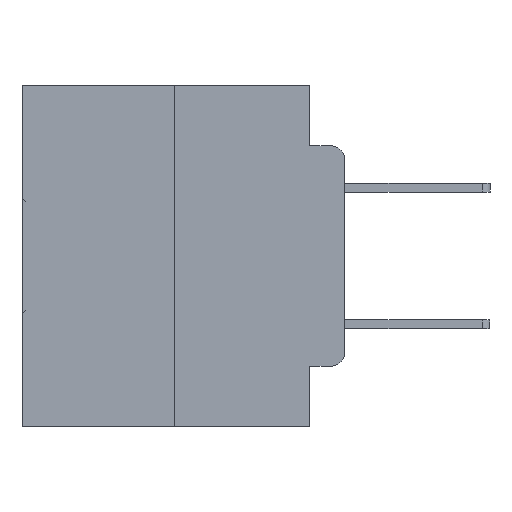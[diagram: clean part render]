
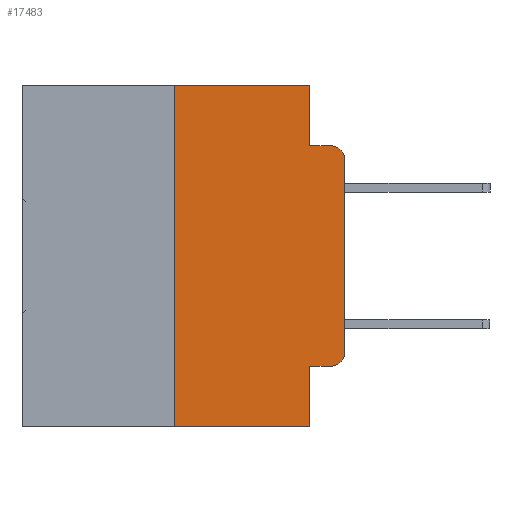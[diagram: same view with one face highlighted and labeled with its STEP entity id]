
A CAD part, left-side view. The second image highlights one B-rep face of the part: STEP entity #17483.
In plain terms, the highlighted planar face has unit normal (-1, 0, 0).
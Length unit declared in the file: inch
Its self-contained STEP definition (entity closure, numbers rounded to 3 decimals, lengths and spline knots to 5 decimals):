
#2217 = ORIENTED_EDGE ( 'NONE', *, *, #10185, .T. ) ;
#2728 = CARTESIAN_POINT ( 'NONE',  ( 0., 0.25, 0. ) ) ;
#2851 = CARTESIAN_POINT ( 'NONE',  ( 0., 0.02, -0.3915 ) ) ;
#2964 = CARTESIAN_POINT ( 'NONE',  ( 0., 0., 0. ) ) ;
#3851 = DIRECTION ( 'NONE',  ( 0., -1., 0. ) ) ;
#4351 = CARTESIAN_POINT ( 'NONE',  ( 0., 0.051, -0.4115 ) ) ;
#4694 = CARTESIAN_POINT ( 'NONE',  ( 0., 0.02, -0.1085 ) ) ;
#4791 = VERTEX_POINT ( 'NONE', #28199 ) ;
#5362 = DIRECTION ( 'NONE',  ( 0., 0., -1. ) ) ;
#5381 = CARTESIAN_POINT ( 'NONE',  ( 0., 0.473, 0. ) ) ;
#6493 = ORIENTED_EDGE ( 'NONE', *, *, #16412, .F. ) ;
#6682 = EDGE_CURVE ( 'NONE', #17174, #18197, #13168, .T. ) ;
#7060 = LINE ( 'NONE', #23543, #14988 ) ;
#7168 = DIRECTION ( 'NONE',  ( 0., 0., -1. ) ) ;
#7213 = LINE ( 'NONE', #28605, #12131 ) ;
#7281 = ORIENTED_EDGE ( 'NONE', *, *, #18904, .F. ) ;
#7459 = LINE ( 'NONE', #27689, #25003 ) ;
#7704 = CARTESIAN_POINT ( 'NONE',  ( 0., 0.051, 0. ) ) ;
#7847 = DIRECTION ( 'NONE',  ( 0., 0., -1. ) ) ;
#8125 = CARTESIAN_POINT ( 'NONE',  ( 0., 0.02, -0.4115 ) ) ;
#8334 = EDGE_CURVE ( 'NONE', #11623, #19923, #7060, .T. ) ;
#9048 = AXIS2_PLACEMENT_3D ( 'NONE', #4694, #21554, #7168 ) ;
#9080 = VERTEX_POINT ( 'NONE', #8125 ) ;
#9521 = DIRECTION ( 'NONE',  ( 0., -1., 0. ) ) ;
#10185 = EDGE_CURVE ( 'NONE', #11623, #18197, #16757, .T. ) ;
#10322 = CARTESIAN_POINT ( 'NONE',  ( 0., 0.051, -0.4115 ) ) ;
#10334 = CARTESIAN_POINT ( 'NONE',  ( 0., 0.25, -0.5 ) ) ;
#10422 = CARTESIAN_POINT ( 'NONE',  ( 0., 0.051, -0.5 ) ) ;
#11623 = VERTEX_POINT ( 'NONE', #10334 ) ;
#12063 = DIRECTION ( 'NONE',  ( 0., 0., -1. ) ) ;
#12115 = CIRCLE ( 'NONE', #26288, 0.02 ) ;
#12131 = VECTOR ( 'NONE', #12063, 39.37008 ) ;
#12577 = PLANE ( 'NONE',  #15588 ) ;
#12725 = DIRECTION ( 'NONE',  ( 0., -1., 0. ) ) ;
#13168 = LINE ( 'NONE', #26592, #18875 ) ;
#13185 = CARTESIAN_POINT ( 'NONE',  ( 0., 0.051, -0.0885 ) ) ;
#14784 = EDGE_CURVE ( 'NONE', #18082, #4791, #7213, .T. ) ;
#14988 = VECTOR ( 'NONE', #23750, 39.37008 ) ;
#15457 = FACE_OUTER_BOUND ( 'NONE', #18785, .T. ) ;
#15588 = AXIS2_PLACEMENT_3D ( 'NONE', #5381, #22221, #7847 ) ;
#15637 = DIRECTION ( 'NONE',  ( 0., -1., 0. ) ) ;
#15769 = LINE ( 'NONE', #10322, #27561 ) ;
#16277 = CIRCLE ( 'NONE', #9048, 0.02 ) ;
#16297 = ORIENTED_EDGE ( 'NONE', *, *, #6682, .F. ) ;
#16412 = EDGE_CURVE ( 'NONE', #4791, #21088, #16545, .T. ) ;
#16545 = LINE ( 'NONE', #13185, #27552 ) ;
#16560 = VERTEX_POINT ( 'NONE', #23332 ) ;
#16757 = LINE ( 'NONE', #21466, #28514 ) ;
#17174 = VERTEX_POINT ( 'NONE', #4351 ) ;
#17429 = DIRECTION ( 'NONE',  ( 0., 0., 1. ) ) ;
#17483 = ADVANCED_FACE ( 'NONE', ( #15457 ), #12577, .F. ) ;
#17898 = VECTOR ( 'NONE', #17429, 39.37008 ) ;
#18082 = VERTEX_POINT ( 'NONE', #7704 ) ;
#18197 = VERTEX_POINT ( 'NONE', #10422 ) ;
#18785 = EDGE_LOOP ( 'NONE', ( #24474, #21164, #6493, #25578, #7281, #20820, #2217, #16297, #22620, #30265 ) ) ;
#18875 = VECTOR ( 'NONE', #19555, 39.37008 ) ;
#18904 = EDGE_CURVE ( 'NONE', #19923, #18082, #7459, .T. ) ;
#19555 = DIRECTION ( 'NONE',  ( 0., 0., -1. ) ) ;
#19833 = DIRECTION ( 'NONE',  ( -1., 0., 0. ) ) ;
#19923 = VERTEX_POINT ( 'NONE', #2728 ) ;
#20820 = ORIENTED_EDGE ( 'NONE', *, *, #8334, .F. ) ;
#21088 = VERTEX_POINT ( 'NONE', #24210 ) ;
#21164 = ORIENTED_EDGE ( 'NONE', *, *, #22774, .T. ) ;
#21232 = VERTEX_POINT ( 'NONE', #29770 ) ;
#21466 = CARTESIAN_POINT ( 'NONE',  ( 0., 0.473, -0.5 ) ) ;
#21554 = DIRECTION ( 'NONE',  ( -1., 0., 0. ) ) ;
#22221 = DIRECTION ( 'NONE',  ( 1., 0., 0. ) ) ;
#22620 = ORIENTED_EDGE ( 'NONE', *, *, #31182, .T. ) ;
#22774 = EDGE_CURVE ( 'NONE', #16560, #21088, #16277, .T. ) ;
#23332 = CARTESIAN_POINT ( 'NONE',  ( 0., 0., -0.1085 ) ) ;
#23543 = CARTESIAN_POINT ( 'NONE',  ( 0., 0.25, 0. ) ) ;
#23750 = DIRECTION ( 'NONE',  ( 0., 0., 1. ) ) ;
#24210 = CARTESIAN_POINT ( 'NONE',  ( 0., 0.02, -0.0885 ) ) ;
#24346 = EDGE_CURVE ( 'NONE', #21232, #16560, #30364, .T. ) ;
#24474 = ORIENTED_EDGE ( 'NONE', *, *, #24346, .T. ) ;
#25003 = VECTOR ( 'NONE', #3851, 39.37008 ) ;
#25578 = ORIENTED_EDGE ( 'NONE', *, *, #14784, .F. ) ;
#26288 = AXIS2_PLACEMENT_3D ( 'NONE', #2851, #19833, #5362 ) ;
#26471 = EDGE_CURVE ( 'NONE', #9080, #21232, #12115, .T. ) ;
#26592 = CARTESIAN_POINT ( 'NONE',  ( 0., 0.051, 0. ) ) ;
#27552 = VECTOR ( 'NONE', #15637, 39.37008 ) ;
#27561 = VECTOR ( 'NONE', #12725, 39.37008 ) ;
#27689 = CARTESIAN_POINT ( 'NONE',  ( 0., 0.473, 0. ) ) ;
#28199 = CARTESIAN_POINT ( 'NONE',  ( 0., 0.051, -0.0885 ) ) ;
#28514 = VECTOR ( 'NONE', #9521, 39.37008 ) ;
#28605 = CARTESIAN_POINT ( 'NONE',  ( 0., 0.051, 0. ) ) ;
#29770 = CARTESIAN_POINT ( 'NONE',  ( 0., 0., -0.3915 ) ) ;
#30265 = ORIENTED_EDGE ( 'NONE', *, *, #26471, .T. ) ;
#30364 = LINE ( 'NONE', #2964, #17898 ) ;
#31182 = EDGE_CURVE ( 'NONE', #17174, #9080, #15769, .T. ) ;
